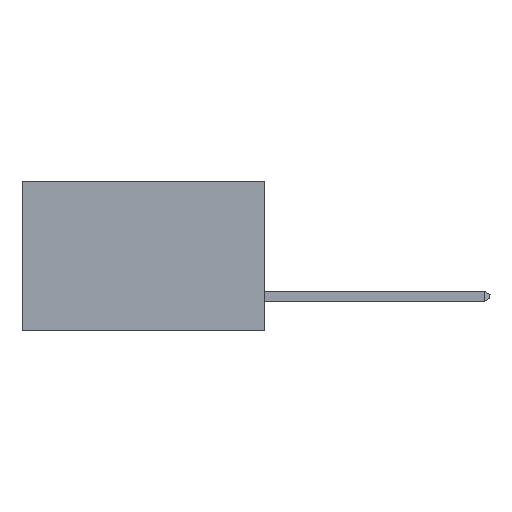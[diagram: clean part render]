
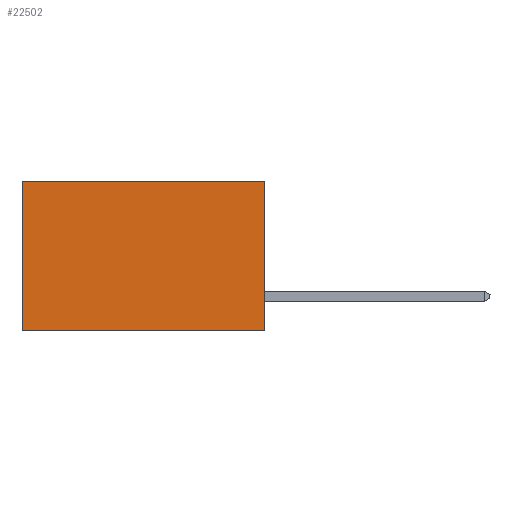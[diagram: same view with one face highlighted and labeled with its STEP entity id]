
A CAD part, left-side view. The second image highlights one B-rep face of the part: STEP entity #22502.
In plain terms, the highlighted planar face has unit normal (-1, 0, 0).
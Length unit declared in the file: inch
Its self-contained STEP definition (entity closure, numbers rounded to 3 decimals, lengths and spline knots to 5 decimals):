
#1185 = CARTESIAN_POINT ( 'NONE',  ( 0.2615, 0., -0.37 ) ) ;
#1186 = VECTOR ( 'NONE', #16980, 39.37008 ) ;
#1996 = DIRECTION ( 'NONE',  ( 1., 0., 0. ) ) ;
#2040 = ORIENTED_EDGE ( 'NONE', *, *, #22443, .T. ) ;
#3235 = DIRECTION ( 'NONE',  ( 0., 1., 0. ) ) ;
#3585 = VECTOR ( 'NONE', #20138, 39.37008 ) ;
#4592 = CARTESIAN_POINT ( 'NONE',  ( 0.2615, 0.6, -0.37 ) ) ;
#5323 = CARTESIAN_POINT ( 'NONE',  ( 0.2615, 0.6, 0. ) ) ;
#6277 = CARTESIAN_POINT ( 'NONE',  ( 0.2615, 0., -0.37 ) ) ;
#6594 = VERTEX_POINT ( 'NONE', #17445 ) ;
#7290 = EDGE_CURVE ( 'NONE', #6594, #8795, #20231, .T. ) ;
#8241 = ORIENTED_EDGE ( 'NONE', *, *, #12310, .T. ) ;
#8707 = CARTESIAN_POINT ( 'NONE',  ( 0.2615, 0.6, -0.37 ) ) ;
#8795 = VERTEX_POINT ( 'NONE', #1185 ) ;
#8937 = DIRECTION ( 'NONE',  ( 0., 0., -1. ) ) ;
#10101 = LINE ( 'NONE', #16652, #1186 ) ;
#10288 = VERTEX_POINT ( 'NONE', #8707 ) ;
#11107 = VECTOR ( 'NONE', #3235, 39.37008 ) ;
#12041 = PLANE ( 'NONE',  #13307 ) ;
#12310 = EDGE_CURVE ( 'NONE', #17178, #10288, #22271, .T. ) ;
#12365 = CARTESIAN_POINT ( 'NONE',  ( 0.2615, 0., -0.37 ) ) ;
#13307 = AXIS2_PLACEMENT_3D ( 'NONE', #12365, #1996, #8937 ) ;
#14397 = VECTOR ( 'NONE', #14856, 39.37008 ) ;
#14856 = DIRECTION ( 'NONE',  ( 0., 0., -1. ) ) ;
#15032 = ORIENTED_EDGE ( 'NONE', *, *, #7290, .F. ) ;
#16652 = CARTESIAN_POINT ( 'NONE',  ( 0.2615, 0., -0.37 ) ) ;
#16980 = DIRECTION ( 'NONE',  ( 0., 1., 0. ) ) ;
#17178 = VERTEX_POINT ( 'NONE', #5323 ) ;
#17445 = CARTESIAN_POINT ( 'NONE',  ( 0.2615, 0., 0. ) ) ;
#17483 = EDGE_CURVE ( 'NONE', #8795, #10288, #10101, .T. ) ;
#18792 = EDGE_LOOP ( 'NONE', ( #8241, #22175, #15032, #2040 ) ) ;
#19340 = LINE ( 'NONE', #20940, #11107 ) ;
#20138 = DIRECTION ( 'NONE',  ( 0., 0., -1. ) ) ;
#20231 = LINE ( 'NONE', #6277, #14397 ) ;
#20940 = CARTESIAN_POINT ( 'NONE',  ( 0.2615, 0., 0. ) ) ;
#22018 = FACE_OUTER_BOUND ( 'NONE', #18792, .T. ) ;
#22175 = ORIENTED_EDGE ( 'NONE', *, *, #17483, .F. ) ;
#22271 = LINE ( 'NONE', #4592, #3585 ) ;
#22443 = EDGE_CURVE ( 'NONE', #6594, #17178, #19340, .T. ) ;
#22502 = ADVANCED_FACE ( 'NONE', ( #22018 ), #12041, .F. ) ;
